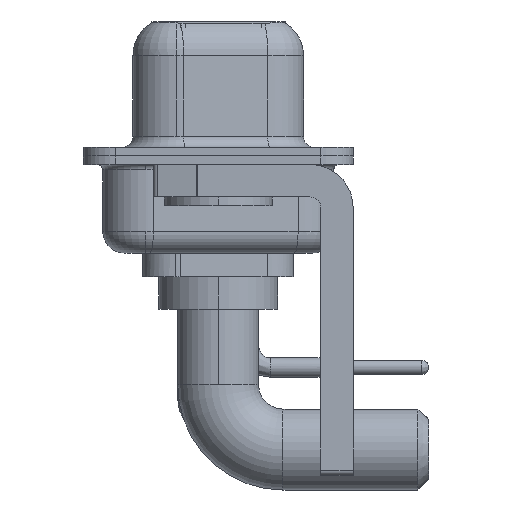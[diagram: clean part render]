
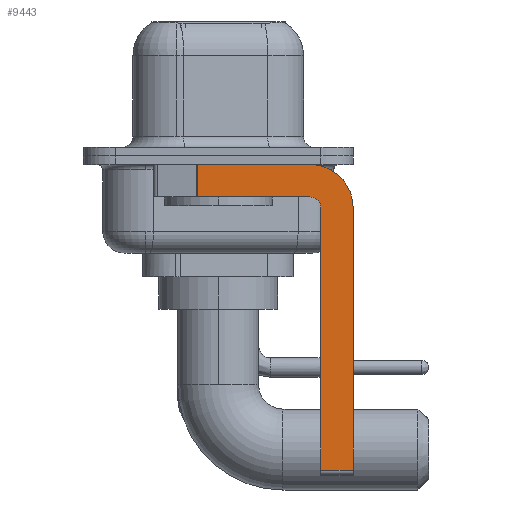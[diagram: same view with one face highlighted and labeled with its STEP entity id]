
A CAD part, left-side view. The second image highlights one B-rep face of the part: STEP entity #9443.
In plain terms, the highlighted planar face has unit normal (-1, 0, 0).
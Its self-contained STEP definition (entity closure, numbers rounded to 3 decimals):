
#711 = CARTESIAN_POINT ( 'NONE',  ( -2.9, -4.25, -14.55 ) ) ;
#1071 = VERTEX_POINT ( 'NONE', #4871 ) ;
#1192 = VERTEX_POINT ( 'NONE', #14859 ) ;
#1223 = DIRECTION ( 'NONE',  ( 0., 0., -1. ) ) ;
#1326 = ORIENTED_EDGE ( 'NONE', *, *, #8949, .F. ) ;
#1415 = VERTEX_POINT ( 'NONE', #11880 ) ;
#1507 = CARTESIAN_POINT ( 'NONE',  ( -2.9, 3., -0.4 ) ) ;
#1604 = DIRECTION ( 'NONE',  ( 1., 0., 0. ) ) ;
#1770 = LINE ( 'NONE', #17544, #11096 ) ;
#1907 = VERTEX_POINT ( 'NONE', #23478 ) ;
#2015 = ORIENTED_EDGE ( 'NONE', *, *, #8883, .F. ) ;
#2679 = VERTEX_POINT ( 'NONE', #18675 ) ;
#3329 = CARTESIAN_POINT ( 'NONE',  ( -2.9, -4.75, -14.8 ) ) ;
#3333 = CIRCLE ( 'NONE', #4957, 0.5 ) ;
#3686 = DIRECTION ( 'NONE',  ( 0., 0., -1. ) ) ;
#4507 = DIRECTION ( 'NONE',  ( -1., 0., 0. ) ) ;
#4713 = DIRECTION ( 'NONE',  ( 0., -1., 0. ) ) ;
#4871 = CARTESIAN_POINT ( 'NONE',  ( -2.9, -4.75, -2.4 ) ) ;
#4896 = CARTESIAN_POINT ( 'NONE',  ( -2.9, -4.25, -0.4 ) ) ;
#4957 = AXIS2_PLACEMENT_3D ( 'NONE', #18607, #4507, #24686 ) ;
#5121 = VECTOR ( 'NONE', #21059, 1000. ) ;
#5494 = LINE ( 'NONE', #21410, #20080 ) ;
#5966 = CARTESIAN_POINT ( 'NONE',  ( -2.9, -4.25, -1.9 ) ) ;
#7173 = CARTESIAN_POINT ( 'NONE',  ( -2.9, -4.25, -2.4 ) ) ;
#7420 = ORIENTED_EDGE ( 'NONE', *, *, #15316, .F. ) ;
#8140 = VERTEX_POINT ( 'NONE', #5966 ) ;
#8290 = VERTEX_POINT ( 'NONE', #4896 ) ;
#8883 = EDGE_CURVE ( 'NONE', #2679, #8290, #13307, .T. ) ;
#8949 = EDGE_CURVE ( 'NONE', #1192, #1071, #14985, .T. ) ;
#9166 = EDGE_CURVE ( 'NONE', #1192, #9491, #10447, .T. ) ;
#9443 = ADVANCED_FACE ( 'NONE', ( #13409 ), #21290, .F. ) ;
#9491 = VERTEX_POINT ( 'NONE', #19466 ) ;
#10447 = LINE ( 'NONE', #711, #10945 ) ;
#10620 = EDGE_CURVE ( 'NONE', #2679, #1907, #5494, .T. ) ;
#10945 = VECTOR ( 'NONE', #4713, 1000. ) ;
#11096 = VECTOR ( 'NONE', #17806, 1000. ) ;
#11456 = CARTESIAN_POINT ( 'NONE',  ( -2.9, -4.25, -2.4 ) ) ;
#11880 = CARTESIAN_POINT ( 'NONE',  ( -2.9, -6.25, -2.4 ) ) ;
#13173 = DIRECTION ( 'NONE',  ( 0., 0., 1. ) ) ;
#13307 = LINE ( 'NONE', #1507, #5121 ) ;
#13409 = FACE_OUTER_BOUND ( 'NONE', #24997, .T. ) ;
#14510 = DIRECTION ( 'NONE',  ( 0., 0., -1. ) ) ;
#14859 = CARTESIAN_POINT ( 'NONE',  ( -2.9, -4.75, -14.55 ) ) ;
#14985 = LINE ( 'NONE', #3329, #24951 ) ;
#15162 = EDGE_CURVE ( 'NONE', #8290, #1415, #16002, .T. ) ;
#15316 = EDGE_CURVE ( 'NONE', #8140, #1907, #23467, .T. ) ;
#15582 = VECTOR ( 'NONE', #17636, 1000. ) ;
#16002 = CIRCLE ( 'NONE', #19715, 2. ) ;
#16240 = EDGE_CURVE ( 'NONE', #1415, #9491, #1770, .T. ) ;
#16605 = ORIENTED_EDGE ( 'NONE', *, *, #15162, .F. ) ;
#17544 = CARTESIAN_POINT ( 'NONE',  ( -2.9, -6.25, -2.4 ) ) ;
#17636 = DIRECTION ( 'NONE',  ( 0., 1., 0. ) ) ;
#17806 = DIRECTION ( 'NONE',  ( 0., 0., -1. ) ) ;
#18081 = EDGE_CURVE ( 'NONE', #1071, #8140, #3333, .T. ) ;
#18607 = CARTESIAN_POINT ( 'NONE',  ( -2.9, -4.25, -2.4 ) ) ;
#18625 = ORIENTED_EDGE ( 'NONE', *, *, #9166, .T. ) ;
#18675 = CARTESIAN_POINT ( 'NONE',  ( -2.9, 0.978, -0.4 ) ) ;
#19466 = CARTESIAN_POINT ( 'NONE',  ( -2.9, -6.25, -14.55 ) ) ;
#19589 = CARTESIAN_POINT ( 'NONE',  ( -2.9, -4.25, -1.9 ) ) ;
#19715 = AXIS2_PLACEMENT_3D ( 'NONE', #7173, #22698, #1223 ) ;
#20028 = AXIS2_PLACEMENT_3D ( 'NONE', #11456, #1604, #14510 ) ;
#20080 = VECTOR ( 'NONE', #3686, 1000. ) ;
#21059 = DIRECTION ( 'NONE',  ( 0., -1., 0. ) ) ;
#21290 = PLANE ( 'NONE',  #20028 ) ;
#21410 = CARTESIAN_POINT ( 'NONE',  ( -2.9, 0.978, -1.9 ) ) ;
#22136 = ORIENTED_EDGE ( 'NONE', *, *, #10620, .T. ) ;
#22387 = ORIENTED_EDGE ( 'NONE', *, *, #18081, .F. ) ;
#22477 = ORIENTED_EDGE ( 'NONE', *, *, #16240, .F. ) ;
#22698 = DIRECTION ( 'NONE',  ( 1., 0., 0. ) ) ;
#23467 = LINE ( 'NONE', #19589, #15582 ) ;
#23478 = CARTESIAN_POINT ( 'NONE',  ( -2.9, 0.978, -1.9 ) ) ;
#24686 = DIRECTION ( 'NONE',  ( 0., 0., 1. ) ) ;
#24951 = VECTOR ( 'NONE', #13173, 1000. ) ;
#24997 = EDGE_LOOP ( 'NONE', ( #2015, #22136, #7420, #22387, #1326, #18625, #22477, #16605 ) ) ;
